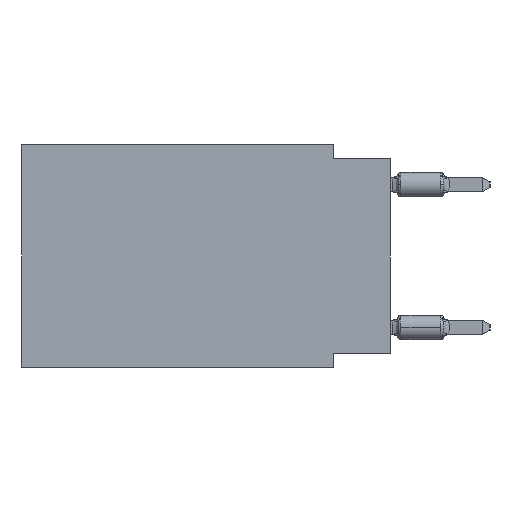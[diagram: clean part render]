
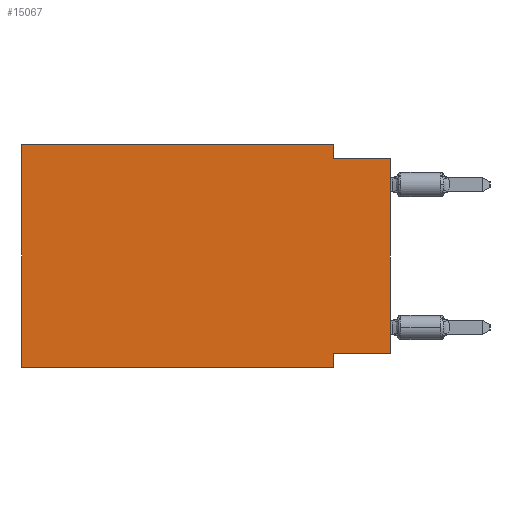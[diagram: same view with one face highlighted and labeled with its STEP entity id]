
A CAD part, left-side view. The second image highlights one B-rep face of the part: STEP entity #15067.
In plain terms, the highlighted planar face has unit normal (-1, 0, 0).
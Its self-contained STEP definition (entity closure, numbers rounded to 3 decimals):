
#92 = EDGE_CURVE ( 'NONE', #14519, #24946, #24369, .T. ) ;
#1319 = DIRECTION ( 'NONE',  ( 0., -1., 0. ) ) ;
#1555 = ORIENTED_EDGE ( 'NONE', *, *, #23181, .F. ) ;
#1564 = VERTEX_POINT ( 'NONE', #2861 ) ;
#1590 = DIRECTION ( 'NONE',  ( 0., 1., 0. ) ) ;
#2148 = CARTESIAN_POINT ( 'NONE',  ( 0., 0., -9.271 ) ) ;
#2861 = CARTESIAN_POINT ( 'NONE',  ( 0., 2.54, -9.271 ) ) ;
#3431 = EDGE_CURVE ( 'NONE', #26315, #30262, #29617, .T. ) ;
#3672 = EDGE_CURVE ( 'NONE', #26825, #11961, #29401, .T. ) ;
#3878 = VECTOR ( 'NONE', #28670, 1000. ) ;
#4452 = VERTEX_POINT ( 'NONE', #16728 ) ;
#4474 = CARTESIAN_POINT ( 'NONE',  ( 0., 0., -0.635 ) ) ;
#4542 = DIRECTION ( 'NONE',  ( 0., -1., 0. ) ) ;
#5203 = DIRECTION ( 'NONE',  ( 0., 0., -1. ) ) ;
#5658 = DIRECTION ( 'NONE',  ( 1., 0., 0. ) ) ;
#6135 = CARTESIAN_POINT ( 'NONE',  ( 0., 16.383, -9.906 ) ) ;
#7559 = PLANE ( 'NONE',  #27959 ) ;
#7996 = CARTESIAN_POINT ( 'NONE',  ( 0., 2.54, 0. ) ) ;
#8018 = ORIENTED_EDGE ( 'NONE', *, *, #15681, .F. ) ;
#8359 = LINE ( 'NONE', #18452, #29443 ) ;
#9194 = VECTOR ( 'NONE', #10963, 1000. ) ;
#9258 = CARTESIAN_POINT ( 'NONE',  ( 0., 2.54, -0.635 ) ) ;
#9847 = CARTESIAN_POINT ( 'NONE',  ( 0., 0., 0. ) ) ;
#10963 = DIRECTION ( 'NONE',  ( 0., 0., 1. ) ) ;
#11076 = EDGE_LOOP ( 'NONE', ( #28207, #27674, #14377, #8018, #15916, #23180, #12471, #1555 ) ) ;
#11961 = VERTEX_POINT ( 'NONE', #18969 ) ;
#12398 = CARTESIAN_POINT ( 'NONE',  ( 0., 2.54, -9.906 ) ) ;
#12471 = ORIENTED_EDGE ( 'NONE', *, *, #29060, .F. ) ;
#13609 = CARTESIAN_POINT ( 'NONE',  ( 0., 16.383, 0. ) ) ;
#13995 = VECTOR ( 'NONE', #14437, 1000. ) ;
#14101 = VECTOR ( 'NONE', #14612, 1000. ) ;
#14377 = ORIENTED_EDGE ( 'NONE', *, *, #3431, .F. ) ;
#14437 = DIRECTION ( 'NONE',  ( 0., 0., 1. ) ) ;
#14519 = VERTEX_POINT ( 'NONE', #2148 ) ;
#14612 = DIRECTION ( 'NONE',  ( 0., 0., -1. ) ) ;
#15067 = ADVANCED_FACE ( 'NONE', ( #29184 ), #7559, .F. ) ;
#15681 = EDGE_CURVE ( 'NONE', #4452, #26315, #20221, .T. ) ;
#15916 = ORIENTED_EDGE ( 'NONE', *, *, #21162, .F. ) ;
#16425 = VECTOR ( 'NONE', #4542, 1000. ) ;
#16728 = CARTESIAN_POINT ( 'NONE',  ( 0., 16.383, 0. ) ) ;
#16820 = EDGE_CURVE ( 'NONE', #30262, #24946, #21101, .T. ) ;
#17182 = CARTESIAN_POINT ( 'NONE',  ( 0., 16.383, 0. ) ) ;
#18200 = CARTESIAN_POINT ( 'NONE',  ( 0., 16.383, 0. ) ) ;
#18418 = CARTESIAN_POINT ( 'NONE',  ( 0., 0., -0.635 ) ) ;
#18452 = CARTESIAN_POINT ( 'NONE',  ( 0., 0., -9.271 ) ) ;
#18969 = CARTESIAN_POINT ( 'NONE',  ( 0., 2.54, -9.906 ) ) ;
#19038 = CARTESIAN_POINT ( 'NONE',  ( 0., 16.383, -9.906 ) ) ;
#20221 = LINE ( 'NONE', #13609, #25455 ) ;
#21101 = LINE ( 'NONE', #18418, #16425 ) ;
#21162 = EDGE_CURVE ( 'NONE', #26825, #4452, #25158, .T. ) ;
#21555 = LINE ( 'NONE', #12398, #14101 ) ;
#23180 = ORIENTED_EDGE ( 'NONE', *, *, #3672, .T. ) ;
#23181 = EDGE_CURVE ( 'NONE', #14519, #1564, #8359, .T. ) ;
#24369 = LINE ( 'NONE', #9847, #13995 ) ;
#24650 = CARTESIAN_POINT ( 'NONE',  ( 0., 2.54, 0. ) ) ;
#24946 = VERTEX_POINT ( 'NONE', #4474 ) ;
#25158 = LINE ( 'NONE', #18200, #9194 ) ;
#25455 = VECTOR ( 'NONE', #1319, 1000. ) ;
#26315 = VERTEX_POINT ( 'NONE', #24650 ) ;
#26825 = VERTEX_POINT ( 'NONE', #6135 ) ;
#27674 = ORIENTED_EDGE ( 'NONE', *, *, #16820, .F. ) ;
#27959 = AXIS2_PLACEMENT_3D ( 'NONE', #17182, #5658, #5203 ) ;
#28207 = ORIENTED_EDGE ( 'NONE', *, *, #92, .T. ) ;
#28263 = VECTOR ( 'NONE', #29938, 1000. ) ;
#28670 = DIRECTION ( 'NONE',  ( 0., -1., 0. ) ) ;
#29060 = EDGE_CURVE ( 'NONE', #1564, #11961, #21555, .T. ) ;
#29184 = FACE_OUTER_BOUND ( 'NONE', #11076, .T. ) ;
#29401 = LINE ( 'NONE', #19038, #3878 ) ;
#29443 = VECTOR ( 'NONE', #1590, 1000. ) ;
#29617 = LINE ( 'NONE', #7996, #28263 ) ;
#29938 = DIRECTION ( 'NONE',  ( 0., 0., -1. ) ) ;
#30262 = VERTEX_POINT ( 'NONE', #9258 ) ;
